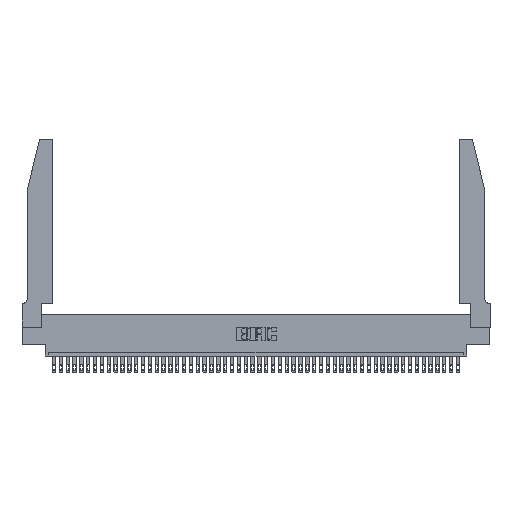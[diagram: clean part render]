
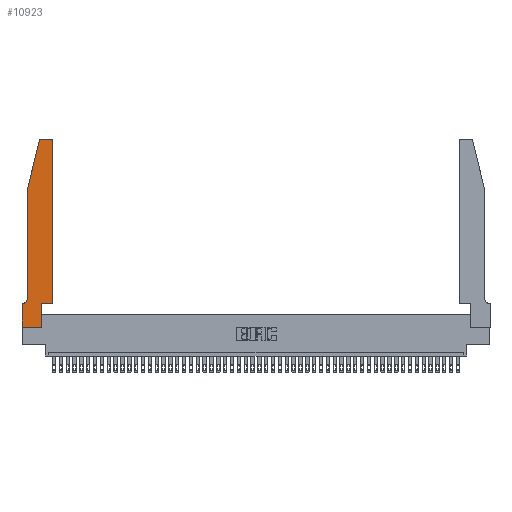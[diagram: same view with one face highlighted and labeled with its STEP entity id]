
A CAD part, top view. The second image highlights one B-rep face of the part: STEP entity #10923.
In plain terms, the highlighted planar face has unit normal (0, 0, 1).
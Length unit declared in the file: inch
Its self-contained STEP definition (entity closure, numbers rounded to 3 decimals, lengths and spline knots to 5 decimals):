
#1030 = CARTESIAN_POINT ( 'NONE',  ( 0.2865, 0.35, 0.37 ) ) ;
#1109 = VERTEX_POINT ( 'NONE', #18765 ) ;
#1112 = CARTESIAN_POINT ( 'NONE',  ( 0.2865, 0.35, 0.37 ) ) ;
#1787 = CARTESIAN_POINT ( 'NONE',  ( 0.0755, 2., 0.37 ) ) ;
#2745 = CIRCLE ( 'NONE', #3716, 0.07 ) ;
#3128 = EDGE_CURVE ( 'NONE', #21953, #38227, #45734, .T. ) ;
#3234 = LINE ( 'NONE', #14340, #41077 ) ;
#3283 = DIRECTION ( 'NONE',  ( 1., 0., 0. ) ) ;
#3716 = AXIS2_PLACEMENT_3D ( 'NONE', #31190, #35359, #38717 ) ;
#3898 = DIRECTION ( 'NONE',  ( 0., 0., 1. ) ) ;
#4462 = CARTESIAN_POINT ( 'NONE',  ( 0.4505, 0.35, 0.37 ) ) ;
#5164 = VERTEX_POINT ( 'NONE', #25357 ) ;
#5286 = CARTESIAN_POINT ( 'NONE',  ( 0.284, 2.72, 0.37 ) ) ;
#6333 = DIRECTION ( 'NONE',  ( -1., 0., 0. ) ) ;
#7379 = ORIENTED_EDGE ( 'NONE', *, *, #3128, .T. ) ;
#7966 = ORIENTED_EDGE ( 'NONE', *, *, #26963, .T. ) ;
#9487 = CARTESIAN_POINT ( 'NONE',  ( 0.4205, 2.75, 0.37 ) ) ;
#10328 = DIRECTION ( 'NONE',  ( 0., 1., 0. ) ) ;
#10923 = ADVANCED_FACE ( 'NONE', ( #36756 ), #37403, .T. ) ;
#10937 = ORIENTED_EDGE ( 'NONE', *, *, #33541, .T. ) ;
#11046 = ORIENTED_EDGE ( 'NONE', *, *, #25918, .T. ) ;
#11298 = LINE ( 'NONE', #42864, #21027 ) ;
#11387 = ORIENTED_EDGE ( 'NONE', *, *, #28723, .T. ) ;
#11828 = VERTEX_POINT ( 'NONE', #26171 ) ;
#12024 = VECTOR ( 'NONE', #12359, 39.37008 ) ;
#12196 = LINE ( 'NONE', #32277, #29948 ) ;
#12359 = DIRECTION ( 'NONE',  ( 1., 0., 0. ) ) ;
#12606 = CARTESIAN_POINT ( 'NONE',  ( 0., 0.35, 0.37 ) ) ;
#12893 = ORIENTED_EDGE ( 'NONE', *, *, #39114, .T. ) ;
#14145 = EDGE_CURVE ( 'NONE', #32294, #11828, #22613, .T. ) ;
#14163 = CARTESIAN_POINT ( 'NONE',  ( 0.2605, 2.75, 0.37 ) ) ;
#14312 = LINE ( 'NONE', #38589, #12024 ) ;
#14340 = CARTESIAN_POINT ( 'NONE',  ( 0.0755, 2., 0.37 ) ) ;
#15204 = AXIS2_PLACEMENT_3D ( 'NONE', #25865, #3898, #3283 ) ;
#15437 = VERTEX_POINT ( 'NONE', #1112 ) ;
#17254 = CARTESIAN_POINT ( 'NONE',  ( 0.0755, 0.42, 0.37 ) ) ;
#18025 = CARTESIAN_POINT ( 'NONE',  ( 0., 0., 0.37 ) ) ;
#18611 = DIRECTION ( 'NONE',  ( 0., -1., 0. ) ) ;
#18765 = CARTESIAN_POINT ( 'NONE',  ( 0.4505, 0.35, 0.37 ) ) ;
#19970 = DIRECTION ( 'NONE',  ( 1., 0., 0. ) ) ;
#21027 = VECTOR ( 'NONE', #10328, 39.37008 ) ;
#21222 = EDGE_CURVE ( 'NONE', #1109, #45167, #11298, .T. ) ;
#21622 = EDGE_CURVE ( 'NONE', #11828, #21953, #3234, .T. ) ;
#21953 = VERTEX_POINT ( 'NONE', #34152 ) ;
#22060 = AXIS2_PLACEMENT_3D ( 'NONE', #33250, #40659, #33397 ) ;
#22191 = VECTOR ( 'NONE', #6333, 39.37008 ) ;
#22613 = CIRCLE ( 'NONE', #28944, 0.03 ) ;
#22806 = ORIENTED_EDGE ( 'NONE', *, *, #43669, .T. ) ;
#23941 = CIRCLE ( 'NONE', #15204, 0.03 ) ;
#24659 = LINE ( 'NONE', #4462, #29188 ) ;
#24753 = VERTEX_POINT ( 'NONE', #12606 ) ;
#25357 = CARTESIAN_POINT ( 'NONE',  ( 0.2865, 0., 0.37 ) ) ;
#25859 = EDGE_CURVE ( 'NONE', #15437, #1109, #24659, .T. ) ;
#25865 = CARTESIAN_POINT ( 'NONE',  ( 0.4205, 2.72, 0.37 ) ) ;
#25918 = EDGE_CURVE ( 'NONE', #42519, #5164, #14312, .T. ) ;
#26171 = CARTESIAN_POINT ( 'NONE',  ( 0.25487, 2.72718, 0.37 ) ) ;
#26963 = EDGE_CURVE ( 'NONE', #45167, #32999, #23941, .T. ) ;
#27832 = VERTEX_POINT ( 'NONE', #43230 ) ;
#28334 = VECTOR ( 'NONE', #18611, 39.37008 ) ;
#28723 = EDGE_CURVE ( 'NONE', #24753, #42519, #29440, .T. ) ;
#28944 = AXIS2_PLACEMENT_3D ( 'NONE', #5286, #42005, #19970 ) ;
#29188 = VECTOR ( 'NONE', #30107, 39.37008 ) ;
#29440 = LINE ( 'NONE', #18025, #28334 ) ;
#29516 = EDGE_CURVE ( 'NONE', #27832, #24753, #12196, .T. ) ;
#29948 = VECTOR ( 'NONE', #36004, 39.37008 ) ;
#29954 = VECTOR ( 'NONE', #41616, 39.37008 ) ;
#30107 = DIRECTION ( 'NONE',  ( 1., 0., 0. ) ) ;
#30191 = VECTOR ( 'NONE', #34801, 39.37008 ) ;
#31190 = CARTESIAN_POINT ( 'NONE',  ( 0.0055, 0.42, 0.37 ) ) ;
#32277 = CARTESIAN_POINT ( 'NONE',  ( 0.0755, 0.35, 0.37 ) ) ;
#32294 = VERTEX_POINT ( 'NONE', #40137 ) ;
#32943 = ORIENTED_EDGE ( 'NONE', *, *, #21622, .T. ) ;
#32999 = VERTEX_POINT ( 'NONE', #9487 ) ;
#33250 = CARTESIAN_POINT ( 'NONE',  ( 0., 0.35, 0.37 ) ) ;
#33397 = DIRECTION ( 'NONE',  ( 1., 0., 0. ) ) ;
#33541 = EDGE_CURVE ( 'NONE', #38227, #27832, #2745, .T. ) ;
#33630 = CARTESIAN_POINT ( 'NONE',  ( 0.4505, 2.72, 0.37 ) ) ;
#34152 = CARTESIAN_POINT ( 'NONE',  ( 0.0755, 2., 0.37 ) ) ;
#34801 = DIRECTION ( 'NONE',  ( 0., -1., 0. ) ) ;
#35359 = DIRECTION ( 'NONE',  ( 0., 0., -1. ) ) ;
#35742 = LINE ( 'NONE', #1030, #29954 ) ;
#36004 = DIRECTION ( 'NONE',  ( -1., 0., 0. ) ) ;
#36678 = ORIENTED_EDGE ( 'NONE', *, *, #21222, .T. ) ;
#36745 = ORIENTED_EDGE ( 'NONE', *, *, #25859, .T. ) ;
#36756 = FACE_OUTER_BOUND ( 'NONE', #39047, .T. ) ;
#37140 = LINE ( 'NONE', #14163, #22191 ) ;
#37403 = PLANE ( 'NONE',  #22060 ) ;
#37681 = CARTESIAN_POINT ( 'NONE',  ( 0., 0., 0.37 ) ) ;
#38227 = VERTEX_POINT ( 'NONE', #17254 ) ;
#38589 = CARTESIAN_POINT ( 'NONE',  ( 0., 0., 0.37 ) ) ;
#38717 = DIRECTION ( 'NONE',  ( -1., 0., 0. ) ) ;
#39047 = EDGE_LOOP ( 'NONE', ( #12893, #46785, #32943, #7379, #10937, #41907, #11387, #11046, #22806, #36745, #36678, #7966 ) ) ;
#39114 = EDGE_CURVE ( 'NONE', #32999, #32294, #37140, .T. ) ;
#40137 = CARTESIAN_POINT ( 'NONE',  ( 0.284, 2.75, 0.37 ) ) ;
#40659 = DIRECTION ( 'NONE',  ( 0., 0., 1. ) ) ;
#41077 = VECTOR ( 'NONE', #46905, 39.37008 ) ;
#41616 = DIRECTION ( 'NONE',  ( 0., 1., 0. ) ) ;
#41907 = ORIENTED_EDGE ( 'NONE', *, *, #29516, .T. ) ;
#42005 = DIRECTION ( 'NONE',  ( 0., 0., 1. ) ) ;
#42519 = VERTEX_POINT ( 'NONE', #37681 ) ;
#42864 = CARTESIAN_POINT ( 'NONE',  ( 0.4505, 0.35, 0.37 ) ) ;
#43230 = CARTESIAN_POINT ( 'NONE',  ( 0.0055, 0.35, 0.37 ) ) ;
#43669 = EDGE_CURVE ( 'NONE', #5164, #15437, #35742, .T. ) ;
#45167 = VERTEX_POINT ( 'NONE', #33630 ) ;
#45734 = LINE ( 'NONE', #1787, #30191 ) ;
#46785 = ORIENTED_EDGE ( 'NONE', *, *, #14145, .T. ) ;
#46905 = DIRECTION ( 'NONE',  ( -0.239, -0.971, 0. ) ) ;
